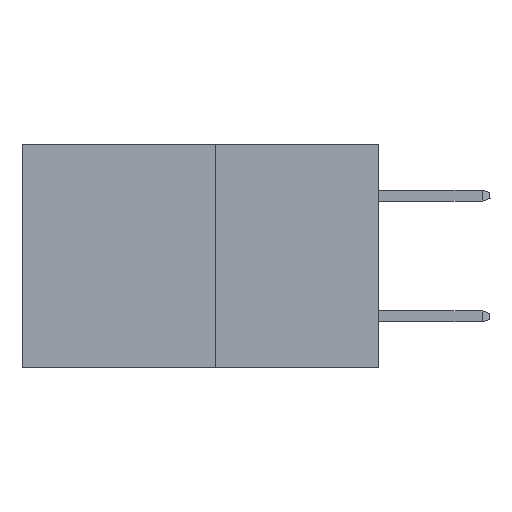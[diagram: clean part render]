
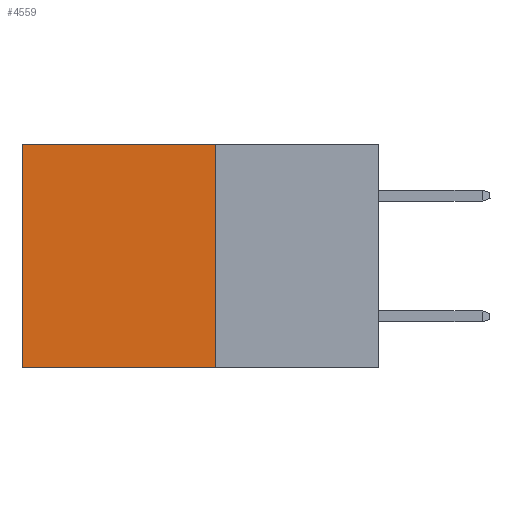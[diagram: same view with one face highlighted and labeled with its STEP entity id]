
A CAD part, left-side view. The second image highlights one B-rep face of the part: STEP entity #4559.
In plain terms, the highlighted planar face has unit normal (-1, 0, 0).
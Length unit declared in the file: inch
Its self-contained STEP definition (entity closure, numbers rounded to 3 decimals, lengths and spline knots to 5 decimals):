
#196 = CARTESIAN_POINT ( 'NONE',  ( 0.277, 0.27, -0.37 ) ) ;
#414 = LINE ( 'NONE', #6802, #3306 ) ;
#748 = DIRECTION ( 'NONE',  ( 0., 1., 0. ) ) ;
#934 = VECTOR ( 'NONE', #8610, 39.37008 ) ;
#1086 = VECTOR ( 'NONE', #748, 39.37008 ) ;
#1488 = EDGE_CURVE ( 'NONE', #10281, #4860, #1597, .T. ) ;
#1597 = LINE ( 'NONE', #9915, #934 ) ;
#1820 = EDGE_LOOP ( 'NONE', ( #12936, #8004, #9454, #12922 ) ) ;
#2104 = EDGE_CURVE ( 'NONE', #2744, #9994, #3942, .T. ) ;
#2548 = DIRECTION ( 'NONE',  ( 0., 0., -1. ) ) ;
#2666 = CARTESIAN_POINT ( 'NONE',  ( 0.277, 0.59, -0.37 ) ) ;
#2744 = VERTEX_POINT ( 'NONE', #4848 ) ;
#3306 = VECTOR ( 'NONE', #6621, 39.37008 ) ;
#3724 = CARTESIAN_POINT ( 'NONE',  ( 0.277, 0.59, 0. ) ) ;
#3942 = LINE ( 'NONE', #196, #1086 ) ;
#4083 = EDGE_CURVE ( 'NONE', #10281, #2744, #414, .T. ) ;
#4377 = VECTOR ( 'NONE', #2548, 39.37008 ) ;
#4559 = ADVANCED_FACE ( 'NONE', ( #7122 ), #12028, .F. ) ;
#4848 = CARTESIAN_POINT ( 'NONE',  ( 0.277, 0.27, -0.37 ) ) ;
#4860 = VERTEX_POINT ( 'NONE', #3724 ) ;
#6621 = DIRECTION ( 'NONE',  ( 0., 0., -1. ) ) ;
#6802 = CARTESIAN_POINT ( 'NONE',  ( 0.277, 0.27, -0.37 ) ) ;
#7122 = FACE_OUTER_BOUND ( 'NONE', #1820, .T. ) ;
#8004 = ORIENTED_EDGE ( 'NONE', *, *, #2104, .F. ) ;
#8571 = EDGE_CURVE ( 'NONE', #4860, #9994, #9981, .T. ) ;
#8610 = DIRECTION ( 'NONE',  ( 0., 1., 0. ) ) ;
#9454 = ORIENTED_EDGE ( 'NONE', *, *, #4083, .F. ) ;
#9915 = CARTESIAN_POINT ( 'NONE',  ( 0.277, 0.27, 0. ) ) ;
#9981 = LINE ( 'NONE', #2666, #4377 ) ;
#9994 = VERTEX_POINT ( 'NONE', #12596 ) ;
#10281 = VERTEX_POINT ( 'NONE', #12064 ) ;
#10433 = AXIS2_PLACEMENT_3D ( 'NONE', #12490, #11978, #11950 ) ;
#11950 = DIRECTION ( 'NONE',  ( 0., 0., -1. ) ) ;
#11978 = DIRECTION ( 'NONE',  ( 1., 0., 0. ) ) ;
#12028 = PLANE ( 'NONE',  #10433 ) ;
#12064 = CARTESIAN_POINT ( 'NONE',  ( 0.277, 0.27, 0. ) ) ;
#12490 = CARTESIAN_POINT ( 'NONE',  ( 0.277, 0.27, -0.37 ) ) ;
#12596 = CARTESIAN_POINT ( 'NONE',  ( 0.277, 0.59, -0.37 ) ) ;
#12922 = ORIENTED_EDGE ( 'NONE', *, *, #1488, .T. ) ;
#12936 = ORIENTED_EDGE ( 'NONE', *, *, #8571, .T. ) ;
